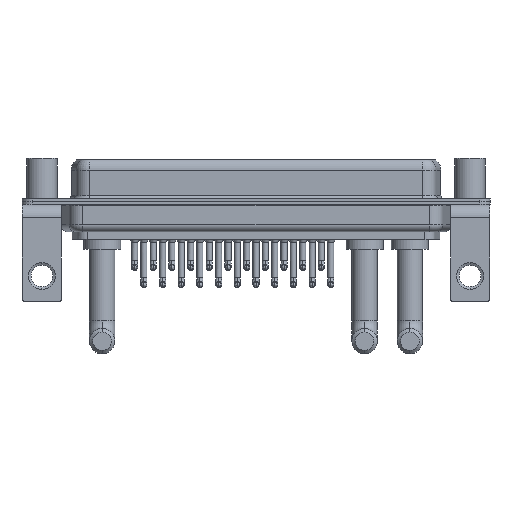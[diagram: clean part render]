
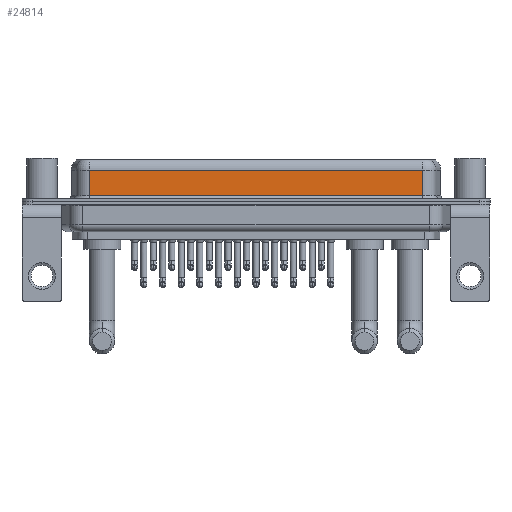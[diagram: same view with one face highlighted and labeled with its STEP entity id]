
A CAD part, front view. The second image highlights one B-rep face of the part: STEP entity #24814.
In plain terms, the highlighted planar face has unit normal (0, -1, 0).
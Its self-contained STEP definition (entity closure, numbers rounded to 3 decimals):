
#2063 = CARTESIAN_POINT ( 'NONE',  ( 56.462, -3.95, 4.65 ) ) ;
#3351 = DIRECTION ( 'NONE',  ( 0., 0., -1. ) ) ;
#3723 = DIRECTION ( 'NONE',  ( 1., 0., 0. ) ) ;
#3860 = CARTESIAN_POINT ( 'NONE',  ( 56.462, -3.95, 0.9 ) ) ;
#3871 = CARTESIAN_POINT ( 'NONE',  ( 7.038, -3.95, 4.65 ) ) ;
#4582 = LINE ( 'NONE', #16840, #5350 ) ;
#4685 = ORIENTED_EDGE ( 'NONE', *, *, #23124, .T. ) ;
#4875 = CARTESIAN_POINT ( 'NONE',  ( 56.462, -3.95, 6.4 ) ) ;
#5350 = VECTOR ( 'NONE', #25107, 1000. ) ;
#6663 = LINE ( 'NONE', #3860, #14158 ) ;
#7191 = VERTEX_POINT ( 'NONE', #19730 ) ;
#9419 = EDGE_LOOP ( 'NONE', ( #24160, #16607, #4685, #25994 ) ) ;
#9766 = DIRECTION ( 'NONE',  ( 0., 1., 0. ) ) ;
#9812 = EDGE_CURVE ( 'NONE', #10156, #10672, #23140, .T. ) ;
#10156 = VERTEX_POINT ( 'NONE', #2063 ) ;
#10165 = FACE_OUTER_BOUND ( 'NONE', #9419, .T. ) ;
#10672 = VERTEX_POINT ( 'NONE', #20539 ) ;
#13476 = CARTESIAN_POINT ( 'NONE',  ( 7.038, -3.95, 6.4 ) ) ;
#14158 = VECTOR ( 'NONE', #3723, 1000. ) ;
#15619 = VERTEX_POINT ( 'NONE', #3871 ) ;
#16010 = PLANE ( 'NONE',  #25224 ) ;
#16182 = EDGE_CURVE ( 'NONE', #10156, #15619, #4582, .T. ) ;
#16267 = VECTOR ( 'NONE', #3351, 1000. ) ;
#16607 = ORIENTED_EDGE ( 'NONE', *, *, #16182, .T. ) ;
#16840 = CARTESIAN_POINT ( 'NONE',  ( 56.462, -3.95, 4.65 ) ) ;
#19111 = DIRECTION ( 'NONE',  ( 0., 0., -1. ) ) ;
#19730 = CARTESIAN_POINT ( 'NONE',  ( 7.038, -3.95, 0.9 ) ) ;
#20151 = CARTESIAN_POINT ( 'NONE',  ( 56.462, -3.95, 6.4 ) ) ;
#20278 = DIRECTION ( 'NONE',  ( 0., 0., 1. ) ) ;
#20539 = CARTESIAN_POINT ( 'NONE',  ( 56.462, -3.95, 0.9 ) ) ;
#23124 = EDGE_CURVE ( 'NONE', #15619, #7191, #23609, .T. ) ;
#23140 = LINE ( 'NONE', #4875, #23418 ) ;
#23418 = VECTOR ( 'NONE', #19111, 1000. ) ;
#23609 = LINE ( 'NONE', #13476, #16267 ) ;
#24160 = ORIENTED_EDGE ( 'NONE', *, *, #9812, .F. ) ;
#24814 = ADVANCED_FACE ( 'NONE', ( #10165 ), #16010, .F. ) ;
#25107 = DIRECTION ( 'NONE',  ( -1., 0., 0. ) ) ;
#25224 = AXIS2_PLACEMENT_3D ( 'NONE', #20151, #9766, #20278 ) ;
#25240 = EDGE_CURVE ( 'NONE', #7191, #10672, #6663, .T. ) ;
#25994 = ORIENTED_EDGE ( 'NONE', *, *, #25240, .T. ) ;
